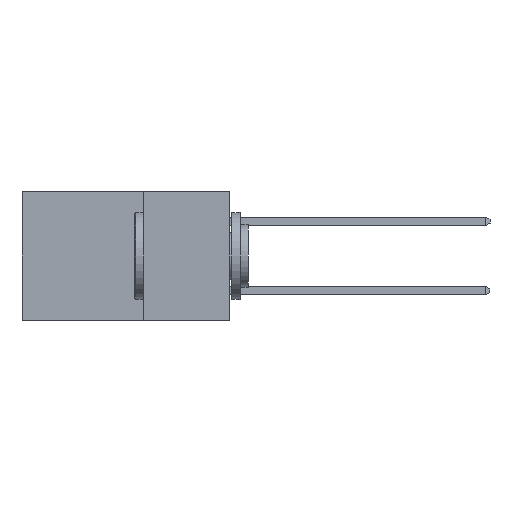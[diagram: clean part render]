
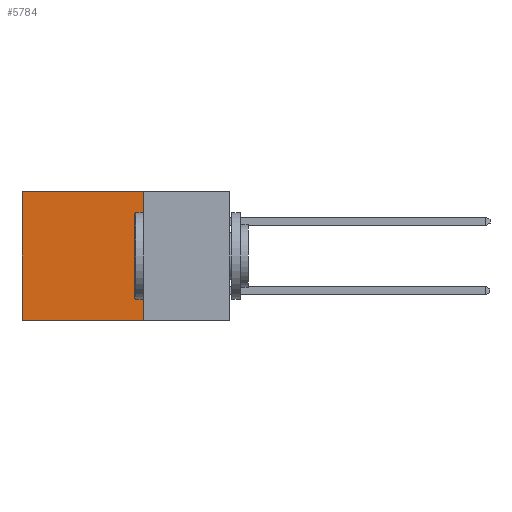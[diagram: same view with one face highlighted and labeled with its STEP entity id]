
A CAD part, left-side view. The second image highlights one B-rep face of the part: STEP entity #5784.
In plain terms, the highlighted planar face has unit normal (-1, 0, 0).
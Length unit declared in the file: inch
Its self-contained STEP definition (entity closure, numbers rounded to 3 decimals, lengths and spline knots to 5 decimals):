
#1409 = ORIENTED_EDGE ( 'NONE', *, *, #11544, .T. ) ;
#1427 = DIRECTION ( 'NONE',  ( 0., 1., 0. ) ) ;
#1513 = ORIENTED_EDGE ( 'NONE', *, *, #8886, .F. ) ;
#1562 = ORIENTED_EDGE ( 'NONE', *, *, #7943, .F. ) ;
#1674 = ORIENTED_EDGE ( 'NONE', *, *, #12189, .T. ) ;
#1853 = VECTOR ( 'NONE', #5953, 39.37008 ) ;
#2114 = VECTOR ( 'NONE', #8093, 39.37008 ) ;
#2883 = EDGE_LOOP ( 'NONE', ( #1409, #1513, #1562, #1674 ) ) ;
#2996 = VERTEX_POINT ( 'NONE', #3079 ) ;
#3079 = CARTESIAN_POINT ( 'NONE',  ( 0.298, 0.25, -0.37 ) ) ;
#3191 = DIRECTION ( 'NONE',  ( 1., 0., 0. ) ) ;
#4290 = VECTOR ( 'NONE', #1427, 39.37008 ) ;
#4924 = LINE ( 'NONE', #9928, #2114 ) ;
#5676 = AXIS2_PLACEMENT_3D ( 'NONE', #10289, #3191, #10780 ) ;
#5742 = CARTESIAN_POINT ( 'NONE',  ( 0.298, 0.6, 0. ) ) ;
#5784 = ADVANCED_FACE ( 'NONE', ( #10014 ), #6268, .F. ) ;
#5887 = VERTEX_POINT ( 'NONE', #12332 ) ;
#5953 = DIRECTION ( 'NONE',  ( 0., 1., 0. ) ) ;
#5996 = VERTEX_POINT ( 'NONE', #8908 ) ;
#6268 = PLANE ( 'NONE',  #5676 ) ;
#6556 = CARTESIAN_POINT ( 'NONE',  ( 0.298, 0.25, -0.37 ) ) ;
#6775 = VERTEX_POINT ( 'NONE', #6828 ) ;
#6828 = CARTESIAN_POINT ( 'NONE',  ( 0.298, 0.6, -0.37 ) ) ;
#7490 = LINE ( 'NONE', #5742, #9676 ) ;
#7943 = EDGE_CURVE ( 'NONE', #5887, #2996, #4924, .T. ) ;
#8093 = DIRECTION ( 'NONE',  ( 0., 0., -1. ) ) ;
#8886 = EDGE_CURVE ( 'NONE', #2996, #6775, #9136, .T. ) ;
#8908 = CARTESIAN_POINT ( 'NONE',  ( 0.298, 0.6, 0. ) ) ;
#9136 = LINE ( 'NONE', #6556, #4290 ) ;
#9507 = LINE ( 'NONE', #9739, #1853 ) ;
#9676 = VECTOR ( 'NONE', #10467, 39.37008 ) ;
#9739 = CARTESIAN_POINT ( 'NONE',  ( 0.298, 0.25, 0. ) ) ;
#9928 = CARTESIAN_POINT ( 'NONE',  ( 0.298, 0.25, 0. ) ) ;
#10014 = FACE_OUTER_BOUND ( 'NONE', #2883, .T. ) ;
#10289 = CARTESIAN_POINT ( 'NONE',  ( 0.298, 0.25, 0. ) ) ;
#10467 = DIRECTION ( 'NONE',  ( 0., 0., -1. ) ) ;
#10780 = DIRECTION ( 'NONE',  ( 0., 0., -1. ) ) ;
#11544 = EDGE_CURVE ( 'NONE', #5996, #6775, #7490, .T. ) ;
#12189 = EDGE_CURVE ( 'NONE', #5887, #5996, #9507, .T. ) ;
#12332 = CARTESIAN_POINT ( 'NONE',  ( 0.298, 0.25, 0. ) ) ;
